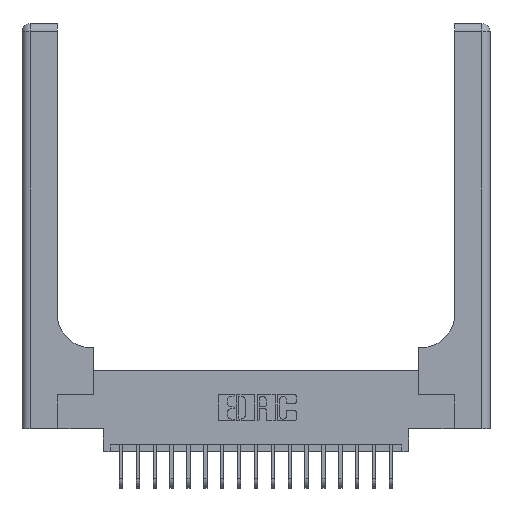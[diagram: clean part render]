
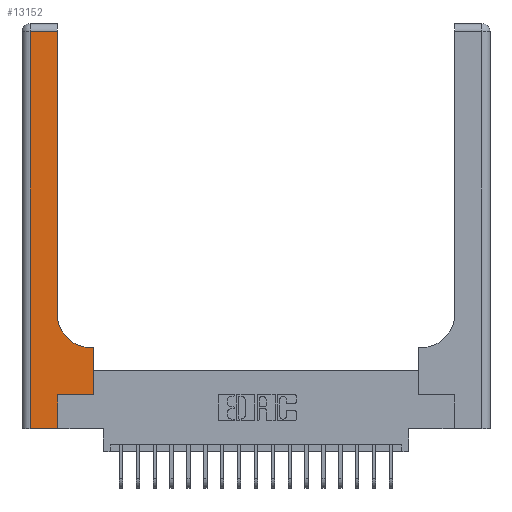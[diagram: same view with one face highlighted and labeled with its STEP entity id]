
A CAD part, top view. The second image highlights one B-rep face of the part: STEP entity #13152.
In plain terms, the highlighted planar face has unit normal (0, 0, 1).
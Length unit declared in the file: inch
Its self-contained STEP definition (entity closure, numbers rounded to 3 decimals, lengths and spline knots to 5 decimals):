
#68 = LINE ( 'NONE', #1215, #13570 ) ;
#633 = DIRECTION ( 'NONE',  ( -1., 0., 0. ) ) ;
#1215 = CARTESIAN_POINT ( 'NONE',  ( 0.528, 0.25, 0.37 ) ) ;
#1758 = LINE ( 'NONE', #9964, #16287 ) ;
#2257 = EDGE_CURVE ( 'NONE', #9342, #18249, #12526, .T. ) ;
#2774 = DIRECTION ( 'NONE',  ( 0., 1., 0. ) ) ;
#2841 = VECTOR ( 'NONE', #16989, 39.37008 ) ;
#2946 = ORIENTED_EDGE ( 'NONE', *, *, #8221, .T. ) ;
#3375 = ORIENTED_EDGE ( 'NONE', *, *, #2257, .T. ) ;
#3534 = VECTOR ( 'NONE', #633, 39.37008 ) ;
#4056 = DIRECTION ( 'NONE',  ( -1., 0., 0. ) ) ;
#4782 = CARTESIAN_POINT ( 'NONE',  ( 0.265, 0.25, 0.37 ) ) ;
#5033 = LINE ( 'NONE', #14515, #6073 ) ;
#5205 = CARTESIAN_POINT ( 'NONE',  ( 0., 3., 0.37 ) ) ;
#5864 = LINE ( 'NONE', #17764, #19403 ) ;
#6073 = VECTOR ( 'NONE', #21317, 39.37008 ) ;
#6474 = EDGE_CURVE ( 'NONE', #12452, #8253, #7955, .T. ) ;
#6510 = LINE ( 'NONE', #12094, #2841 ) ;
#6627 = LINE ( 'NONE', #4782, #16788 ) ;
#6779 = ORIENTED_EDGE ( 'NONE', *, *, #12999, .T. ) ;
#7063 = AXIS2_PLACEMENT_3D ( 'NONE', #15041, #19932, #18159 ) ;
#7116 = CARTESIAN_POINT ( 'NONE',  ( 0.265, 0.25, 0.37 ) ) ;
#7154 = CARTESIAN_POINT ( 'NONE',  ( 0.26, 0.6, 0.37 ) ) ;
#7457 = EDGE_CURVE ( 'NONE', #13189, #9342, #7912, .T. ) ;
#7571 = EDGE_CURVE ( 'NONE', #18249, #12452, #5864, .T. ) ;
#7617 = VERTEX_POINT ( 'NONE', #14327 ) ;
#7912 = LINE ( 'NONE', #7154, #3534 ) ;
#7955 = LINE ( 'NONE', #21214, #9792 ) ;
#8221 = EDGE_CURVE ( 'NONE', #19043, #7617, #6627, .T. ) ;
#8253 = VERTEX_POINT ( 'NONE', #19946 ) ;
#8379 = ORIENTED_EDGE ( 'NONE', *, *, #9920, .T. ) ;
#9129 = CARTESIAN_POINT ( 'NONE',  ( 0.51, 0.6, 0.37 ) ) ;
#9342 = VERTEX_POINT ( 'NONE', #9129 ) ;
#9792 = VECTOR ( 'NONE', #19506, 39.37008 ) ;
#9920 = EDGE_CURVE ( 'NONE', #7617, #13189, #68, .T. ) ;
#9964 = CARTESIAN_POINT ( 'NONE',  ( 0.06, 3., 0.37 ) ) ;
#10650 = DIRECTION ( 'NONE',  ( 0., 0., -1. ) ) ;
#11024 = CARTESIAN_POINT ( 'NONE',  ( 0.26, 0.85, 0.37 ) ) ;
#11133 = EDGE_LOOP ( 'NONE', ( #12240, #21125, #14703, #16605, #6779, #2946, #8379, #12854, #3375 ) ) ;
#11257 = FACE_OUTER_BOUND ( 'NONE', #11133, .T. ) ;
#11545 = DIRECTION ( 'NONE',  ( 1., 0., 0. ) ) ;
#12094 = CARTESIAN_POINT ( 'NONE',  ( 0., 0., 0.37 ) ) ;
#12240 = ORIENTED_EDGE ( 'NONE', *, *, #7571, .T. ) ;
#12452 = VERTEX_POINT ( 'NONE', #18713 ) ;
#12526 = CIRCLE ( 'NONE', #7063, 0.25 ) ;
#12854 = ORIENTED_EDGE ( 'NONE', *, *, #7457, .T. ) ;
#12999 = EDGE_CURVE ( 'NONE', #15131, #19043, #5033, .T. ) ;
#13152 = ADVANCED_FACE ( 'NONE', ( #11257 ), #15195, .F. ) ;
#13189 = VERTEX_POINT ( 'NONE', #15694 ) ;
#13570 = VECTOR ( 'NONE', #20654, 39.37008 ) ;
#13766 = VERTEX_POINT ( 'NONE', #19600 ) ;
#14327 = CARTESIAN_POINT ( 'NONE',  ( 0.528, 0.25, 0.37 ) ) ;
#14515 = CARTESIAN_POINT ( 'NONE',  ( 0.265, 0., 0.37 ) ) ;
#14703 = ORIENTED_EDGE ( 'NONE', *, *, #17728, .T. ) ;
#15041 = CARTESIAN_POINT ( 'NONE',  ( 0.51, 0.85, 0.37 ) ) ;
#15131 = VERTEX_POINT ( 'NONE', #16639 ) ;
#15195 = PLANE ( 'NONE',  #19902 ) ;
#15694 = CARTESIAN_POINT ( 'NONE',  ( 0.528, 0.6, 0.37 ) ) ;
#16287 = VECTOR ( 'NONE', #17956, 39.37008 ) ;
#16605 = ORIENTED_EDGE ( 'NONE', *, *, #20458, .T. ) ;
#16639 = CARTESIAN_POINT ( 'NONE',  ( 0.265, 0., 0.37 ) ) ;
#16788 = VECTOR ( 'NONE', #11545, 39.37008 ) ;
#16989 = DIRECTION ( 'NONE',  ( 1., 0., 0. ) ) ;
#17728 = EDGE_CURVE ( 'NONE', #8253, #13766, #1758, .T. ) ;
#17764 = CARTESIAN_POINT ( 'NONE',  ( 0.26, 3., 0.37 ) ) ;
#17956 = DIRECTION ( 'NONE',  ( 0., -1., 0. ) ) ;
#18159 = DIRECTION ( 'NONE',  ( 1., 0., 0. ) ) ;
#18249 = VERTEX_POINT ( 'NONE', #11024 ) ;
#18713 = CARTESIAN_POINT ( 'NONE',  ( 0.26, 2.94, 0.37 ) ) ;
#19043 = VERTEX_POINT ( 'NONE', #7116 ) ;
#19403 = VECTOR ( 'NONE', #2774, 39.37008 ) ;
#19506 = DIRECTION ( 'NONE',  ( -1., 0., 0. ) ) ;
#19600 = CARTESIAN_POINT ( 'NONE',  ( 0.06, 0., 0.37 ) ) ;
#19902 = AXIS2_PLACEMENT_3D ( 'NONE', #5205, #10650, #4056 ) ;
#19932 = DIRECTION ( 'NONE',  ( 0., 0., -1. ) ) ;
#19946 = CARTESIAN_POINT ( 'NONE',  ( 0.06, 2.94, 0.37 ) ) ;
#20458 = EDGE_CURVE ( 'NONE', #13766, #15131, #6510, .T. ) ;
#20654 = DIRECTION ( 'NONE',  ( 0., 1., 0. ) ) ;
#21125 = ORIENTED_EDGE ( 'NONE', *, *, #6474, .T. ) ;
#21214 = CARTESIAN_POINT ( 'NONE',  ( 0., 2.94, 0.37 ) ) ;
#21317 = DIRECTION ( 'NONE',  ( 0., 1., 0. ) ) ;
